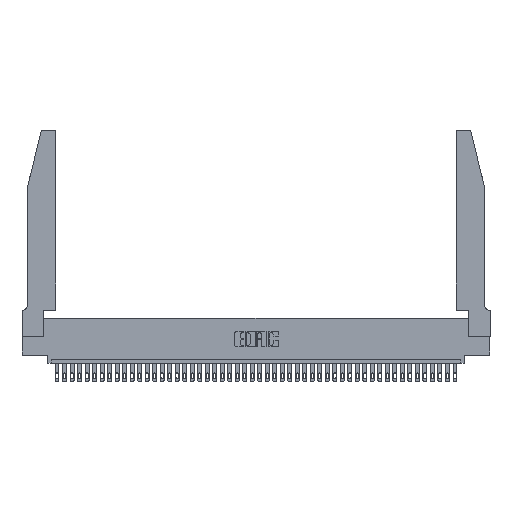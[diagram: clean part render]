
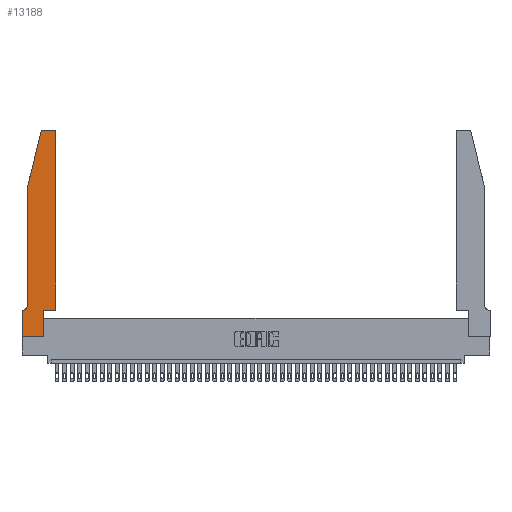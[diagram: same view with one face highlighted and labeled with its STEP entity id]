
A CAD part, top view. The second image highlights one B-rep face of the part: STEP entity #13188.
In plain terms, the highlighted planar face has unit normal (0, 0, 1).
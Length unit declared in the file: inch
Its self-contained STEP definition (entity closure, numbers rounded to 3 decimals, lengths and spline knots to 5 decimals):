
#1289 = ORIENTED_EDGE ( 'NONE', *, *, #16960, .T. ) ;
#1450 = DIRECTION ( 'NONE',  ( 1., 0., 0. ) ) ;
#1522 = AXIS2_PLACEMENT_3D ( 'NONE', #22251, #18873, #2408 ) ;
#1537 = CARTESIAN_POINT ( 'NONE',  ( 0.0055, 0.35, 0.37 ) ) ;
#2001 = AXIS2_PLACEMENT_3D ( 'NONE', #14696, #41707, #24726 ) ;
#2245 = DIRECTION ( 'NONE',  ( -1., 0., 0. ) ) ;
#2408 = DIRECTION ( 'NONE',  ( 1., 0., 0. ) ) ;
#2550 = DIRECTION ( 'NONE',  ( -1., 0., 0. ) ) ;
#2785 = DIRECTION ( 'NONE',  ( 0., 1., 0. ) ) ;
#2790 = VERTEX_POINT ( 'NONE', #33906 ) ;
#3474 = CIRCLE ( 'NONE', #1522, 0.03 ) ;
#3729 = EDGE_CURVE ( 'NONE', #10468, #36678, #19468, .T. ) ;
#4102 = VERTEX_POINT ( 'NONE', #37205 ) ;
#4452 = ORIENTED_EDGE ( 'NONE', *, *, #38069, .T. ) ;
#5628 = LINE ( 'NONE', #34343, #20934 ) ;
#6746 = VECTOR ( 'NONE', #31021, 39.37008 ) ;
#7012 = CARTESIAN_POINT ( 'NONE',  ( 0.4205, 2.75, 0.37 ) ) ;
#7917 = VECTOR ( 'NONE', #17302, 39.37008 ) ;
#7999 = EDGE_CURVE ( 'NONE', #35827, #27097, #21872, .T. ) ;
#9396 = VECTOR ( 'NONE', #1450, 39.37008 ) ;
#9577 = CARTESIAN_POINT ( 'NONE',  ( 0.2865, 0., 0.37 ) ) ;
#10468 = VERTEX_POINT ( 'NONE', #12713 ) ;
#11234 = CARTESIAN_POINT ( 'NONE',  ( 0.4505, 0.35, 0.37 ) ) ;
#11455 = CARTESIAN_POINT ( 'NONE',  ( 0.0055, 0.42, 0.37 ) ) ;
#12095 = LINE ( 'NONE', #35933, #6746 ) ;
#12218 = ORIENTED_EDGE ( 'NONE', *, *, #3729, .T. ) ;
#12713 = CARTESIAN_POINT ( 'NONE',  ( 0.2865, 0.35, 0.37 ) ) ;
#13188 = ADVANCED_FACE ( 'NONE', ( #18904 ), #35008, .T. ) ;
#13210 = AXIS2_PLACEMENT_3D ( 'NONE', #11455, #28155, #28298 ) ;
#13271 = EDGE_CURVE ( 'NONE', #2790, #38228, #12095, .T. ) ;
#14696 = CARTESIAN_POINT ( 'NONE',  ( 0.4205, 2.72, 0.37 ) ) ;
#16281 = LINE ( 'NONE', #41526, #31009 ) ;
#16626 = VERTEX_POINT ( 'NONE', #39294 ) ;
#16960 = EDGE_CURVE ( 'NONE', #4102, #16626, #25933, .T. ) ;
#17302 = DIRECTION ( 'NONE',  ( 0., -1., 0. ) ) ;
#17379 = ORIENTED_EDGE ( 'NONE', *, *, #20825, .T. ) ;
#17889 = CARTESIAN_POINT ( 'NONE',  ( 0., 0.35, 0.37 ) ) ;
#17924 = DIRECTION ( 'NONE',  ( 1., 0., 0. ) ) ;
#18238 = DIRECTION ( 'NONE',  ( 0., 1., 0. ) ) ;
#18873 = DIRECTION ( 'NONE',  ( 0., 0., 1. ) ) ;
#18904 = FACE_OUTER_BOUND ( 'NONE', #31197, .T. ) ;
#18913 = CARTESIAN_POINT ( 'NONE',  ( 0.284, 2.75, 0.37 ) ) ;
#19468 = LINE ( 'NONE', #41395, #9396 ) ;
#19955 = ORIENTED_EDGE ( 'NONE', *, *, #7999, .T. ) ;
#20197 = LINE ( 'NONE', #35832, #36584 ) ;
#20342 = EDGE_CURVE ( 'NONE', #33394, #26969, #36004, .T. ) ;
#20825 = EDGE_CURVE ( 'NONE', #38228, #33394, #22278, .T. ) ;
#20934 = VECTOR ( 'NONE', #2785, 39.37008 ) ;
#21153 = CARTESIAN_POINT ( 'NONE',  ( 0.0755, 2., 0.37 ) ) ;
#21872 = LINE ( 'NONE', #22244, #40877 ) ;
#22244 = CARTESIAN_POINT ( 'NONE',  ( 0.2605, 2.75, 0.37 ) ) ;
#22251 = CARTESIAN_POINT ( 'NONE',  ( 0.284, 2.72, 0.37 ) ) ;
#22278 = LINE ( 'NONE', #21153, #25949 ) ;
#22996 = VERTEX_POINT ( 'NONE', #36511 ) ;
#23074 = EDGE_CURVE ( 'NONE', #27175, #10468, #5628, .T. ) ;
#24268 = ORIENTED_EDGE ( 'NONE', *, *, #13271, .T. ) ;
#24720 = ORIENTED_EDGE ( 'NONE', *, *, #27416, .T. ) ;
#24726 = DIRECTION ( 'NONE',  ( 1., 0., 0. ) ) ;
#25933 = LINE ( 'NONE', #27592, #7917 ) ;
#25949 = VECTOR ( 'NONE', #31198, 39.37008 ) ;
#26403 = VECTOR ( 'NONE', #17924, 39.37008 ) ;
#26421 = ORIENTED_EDGE ( 'NONE', *, *, #31887, .T. ) ;
#26969 = VERTEX_POINT ( 'NONE', #1537 ) ;
#27097 = VERTEX_POINT ( 'NONE', #18913 ) ;
#27175 = VERTEX_POINT ( 'NONE', #9577 ) ;
#27416 = EDGE_CURVE ( 'NONE', #22996, #35827, #34766, .T. ) ;
#27592 = CARTESIAN_POINT ( 'NONE',  ( 0., 0., 0.37 ) ) ;
#27948 = CARTESIAN_POINT ( 'NONE',  ( 0., 0., 0.37 ) ) ;
#28070 = DIRECTION ( 'NONE',  ( 0., 0., 1. ) ) ;
#28155 = DIRECTION ( 'NONE',  ( 0., 0., -1. ) ) ;
#28298 = DIRECTION ( 'NONE',  ( -1., 0., 0. ) ) ;
#29288 = CARTESIAN_POINT ( 'NONE',  ( 0.0755, 2., 0.37 ) ) ;
#31009 = VECTOR ( 'NONE', #18238, 39.37008 ) ;
#31021 = DIRECTION ( 'NONE',  ( -0.239, -0.971, 0. ) ) ;
#31197 = EDGE_LOOP ( 'NONE', ( #19955, #26421, #24268, #17379, #40446, #40406, #1289, #4452, #34772, #12218, #40963, #24720 ) ) ;
#31198 = DIRECTION ( 'NONE',  ( 0., -1., 0. ) ) ;
#31455 = DIRECTION ( 'NONE',  ( 1., 0., 0. ) ) ;
#31887 = EDGE_CURVE ( 'NONE', #27097, #2790, #3474, .T. ) ;
#31953 = EDGE_CURVE ( 'NONE', #26969, #4102, #20197, .T. ) ;
#32311 = AXIS2_PLACEMENT_3D ( 'NONE', #17889, #28070, #31455 ) ;
#33394 = VERTEX_POINT ( 'NONE', #40144 ) ;
#33906 = CARTESIAN_POINT ( 'NONE',  ( 0.25487, 2.72718, 0.37 ) ) ;
#34343 = CARTESIAN_POINT ( 'NONE',  ( 0.2865, 0.35, 0.37 ) ) ;
#34766 = CIRCLE ( 'NONE', #2001, 0.03 ) ;
#34772 = ORIENTED_EDGE ( 'NONE', *, *, #23074, .T. ) ;
#35008 = PLANE ( 'NONE',  #32311 ) ;
#35397 = LINE ( 'NONE', #27948, #26403 ) ;
#35827 = VERTEX_POINT ( 'NONE', #7012 ) ;
#35832 = CARTESIAN_POINT ( 'NONE',  ( 0.0755, 0.35, 0.37 ) ) ;
#35933 = CARTESIAN_POINT ( 'NONE',  ( 0.0755, 2., 0.37 ) ) ;
#36004 = CIRCLE ( 'NONE', #13210, 0.07 ) ;
#36511 = CARTESIAN_POINT ( 'NONE',  ( 0.4505, 2.72, 0.37 ) ) ;
#36584 = VECTOR ( 'NONE', #2550, 39.37008 ) ;
#36678 = VERTEX_POINT ( 'NONE', #11234 ) ;
#37205 = CARTESIAN_POINT ( 'NONE',  ( 0., 0.35, 0.37 ) ) ;
#38069 = EDGE_CURVE ( 'NONE', #16626, #27175, #35397, .T. ) ;
#38228 = VERTEX_POINT ( 'NONE', #29288 ) ;
#39294 = CARTESIAN_POINT ( 'NONE',  ( 0., 0., 0.37 ) ) ;
#40144 = CARTESIAN_POINT ( 'NONE',  ( 0.0755, 0.42, 0.37 ) ) ;
#40406 = ORIENTED_EDGE ( 'NONE', *, *, #31953, .T. ) ;
#40446 = ORIENTED_EDGE ( 'NONE', *, *, #20342, .T. ) ;
#40877 = VECTOR ( 'NONE', #2245, 39.37008 ) ;
#40963 = ORIENTED_EDGE ( 'NONE', *, *, #42458, .T. ) ;
#41395 = CARTESIAN_POINT ( 'NONE',  ( 0.4505, 0.35, 0.37 ) ) ;
#41526 = CARTESIAN_POINT ( 'NONE',  ( 0.4505, 0.35, 0.37 ) ) ;
#41707 = DIRECTION ( 'NONE',  ( 0., 0., 1. ) ) ;
#42458 = EDGE_CURVE ( 'NONE', #36678, #22996, #16281, .T. ) ;
